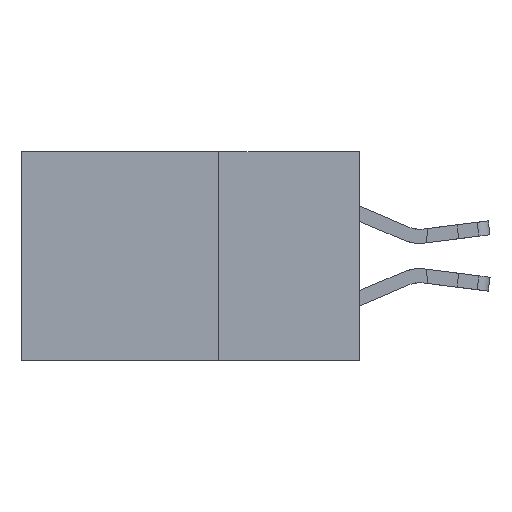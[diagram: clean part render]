
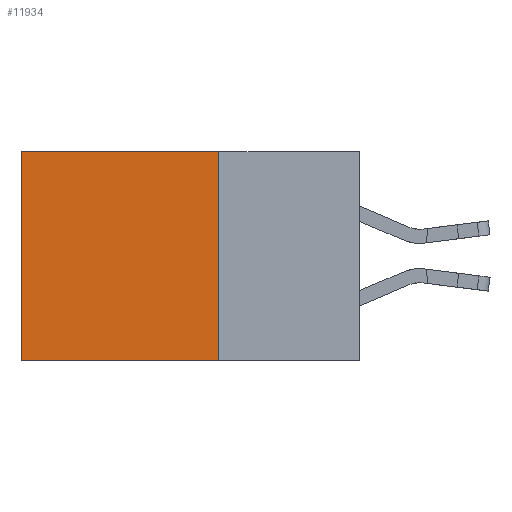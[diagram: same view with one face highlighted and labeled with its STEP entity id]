
A CAD part, left-side view. The second image highlights one B-rep face of the part: STEP entity #11934.
In plain terms, the highlighted planar face has unit normal (-1, 0, 0).
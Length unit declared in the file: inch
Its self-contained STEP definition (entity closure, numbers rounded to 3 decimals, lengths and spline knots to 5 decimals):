
#425 = DIRECTION ( 'NONE',  ( 0., 0., -1. ) ) ;
#1120 = DIRECTION ( 'NONE',  ( 1., 0., 0. ) ) ;
#1285 = ORIENTED_EDGE ( 'NONE', *, *, #15490, .F. ) ;
#2791 = ORIENTED_EDGE ( 'NONE', *, *, #9627, .F. ) ;
#2917 = ORIENTED_EDGE ( 'NONE', *, *, #16502, .T. ) ;
#3415 = VECTOR ( 'NONE', #425, 39.37008 ) ;
#3542 = CARTESIAN_POINT ( 'NONE',  ( 0.2875, 0.25, 0. ) ) ;
#3569 = CARTESIAN_POINT ( 'NONE',  ( 0.2875, 0.6, 0. ) ) ;
#3578 = CARTESIAN_POINT ( 'NONE',  ( 0.2875, 0.6, -0.37 ) ) ;
#4173 = FACE_OUTER_BOUND ( 'NONE', #15795, .T. ) ;
#4897 = CARTESIAN_POINT ( 'NONE',  ( 0.2875, 0.25, 0. ) ) ;
#6536 = CARTESIAN_POINT ( 'NONE',  ( 0.2875, 0.25, 0. ) ) ;
#7702 = AXIS2_PLACEMENT_3D ( 'NONE', #4897, #1120, #10300 ) ;
#8244 = CARTESIAN_POINT ( 'NONE',  ( 0.2875, 0.25, 0. ) ) ;
#8543 = ORIENTED_EDGE ( 'NONE', *, *, #12029, .T. ) ;
#8708 = LINE ( 'NONE', #6536, #9689 ) ;
#8736 = VECTOR ( 'NONE', #12738, 39.37008 ) ;
#9526 = VECTOR ( 'NONE', #12468, 39.37008 ) ;
#9627 = EDGE_CURVE ( 'NONE', #14312, #10258, #11196, .T. ) ;
#9689 = VECTOR ( 'NONE', #15689, 39.37008 ) ;
#10258 = VERTEX_POINT ( 'NONE', #3578 ) ;
#10300 = DIRECTION ( 'NONE',  ( 0., 0., -1. ) ) ;
#10860 = VERTEX_POINT ( 'NONE', #13214 ) ;
#11196 = LINE ( 'NONE', #16378, #9526 ) ;
#11216 = LINE ( 'NONE', #8244, #3415 ) ;
#11417 = PLANE ( 'NONE',  #7702 ) ;
#11934 = ADVANCED_FACE ( 'NONE', ( #4173 ), #11417, .F. ) ;
#12029 = EDGE_CURVE ( 'NONE', #12551, #10860, #8708, .T. ) ;
#12468 = DIRECTION ( 'NONE',  ( 0., 1., 0. ) ) ;
#12551 = VERTEX_POINT ( 'NONE', #3542 ) ;
#12738 = DIRECTION ( 'NONE',  ( 0., 0., -1. ) ) ;
#13019 = LINE ( 'NONE', #3569, #8736 ) ;
#13214 = CARTESIAN_POINT ( 'NONE',  ( 0.2875, 0.6, 0. ) ) ;
#14312 = VERTEX_POINT ( 'NONE', #15856 ) ;
#15490 = EDGE_CURVE ( 'NONE', #12551, #14312, #11216, .T. ) ;
#15689 = DIRECTION ( 'NONE',  ( 0., 1., 0. ) ) ;
#15795 = EDGE_LOOP ( 'NONE', ( #2917, #2791, #1285, #8543 ) ) ;
#15856 = CARTESIAN_POINT ( 'NONE',  ( 0.2875, 0.25, -0.37 ) ) ;
#16378 = CARTESIAN_POINT ( 'NONE',  ( 0.2875, 0.25, -0.37 ) ) ;
#16502 = EDGE_CURVE ( 'NONE', #10860, #10258, #13019, .T. ) ;
